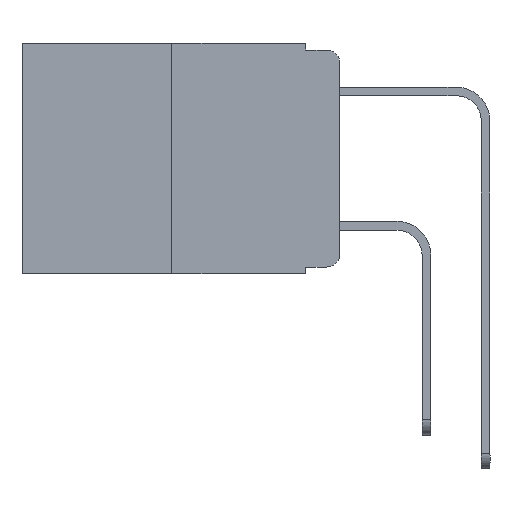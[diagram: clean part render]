
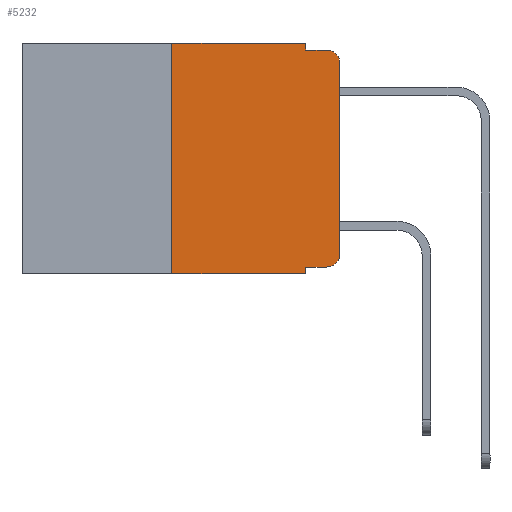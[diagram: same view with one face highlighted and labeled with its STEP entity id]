
A CAD part, left-side view. The second image highlights one B-rep face of the part: STEP entity #5232.
In plain terms, the highlighted planar face has unit normal (-1, 0, 0).
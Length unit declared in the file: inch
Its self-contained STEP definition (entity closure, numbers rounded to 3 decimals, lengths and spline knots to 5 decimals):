
#490 = AXIS2_PLACEMENT_3D ( 'NONE', #6727, #19759, #14586 ) ;
#1292 = VECTOR ( 'NONE', #14065, 39.37008 ) ;
#1585 = CARTESIAN_POINT ( 'NONE',  ( 0., 0.473, -0.343 ) ) ;
#1588 = CARTESIAN_POINT ( 'NONE',  ( 0., 0.25, 0. ) ) ;
#2134 = CARTESIAN_POINT ( 'NONE',  ( 0., 0., 0. ) ) ;
#2191 = EDGE_CURVE ( 'NONE', #2235, #18027, #21104, .T. ) ;
#2235 = VERTEX_POINT ( 'NONE', #5499 ) ;
#2695 = DIRECTION ( 'NONE',  ( 0., 0., 1. ) ) ;
#2850 = LINE ( 'NONE', #12035, #19151 ) ;
#2946 = PLANE ( 'NONE',  #490 ) ;
#3250 = VERTEX_POINT ( 'NONE', #4973 ) ;
#3470 = EDGE_CURVE ( 'NONE', #22289, #11486, #19493, .T. ) ;
#3497 = DIRECTION ( 'NONE',  ( -1., 0., 0. ) ) ;
#3571 = CARTESIAN_POINT ( 'NONE',  ( 0., 0.051, -0.333 ) ) ;
#4194 = CARTESIAN_POINT ( 'NONE',  ( 0., 0.02, -0.313 ) ) ;
#4538 = CARTESIAN_POINT ( 'NONE',  ( 0., 0.25, 0. ) ) ;
#4973 = CARTESIAN_POINT ( 'NONE',  ( 0., 0.051, 0. ) ) ;
#5232 = ADVANCED_FACE ( 'NONE', ( #16016 ), #2946, .F. ) ;
#5252 = LINE ( 'NONE', #21573, #1292 ) ;
#5464 = DIRECTION ( 'NONE',  ( 0., 0., -1. ) ) ;
#5499 = CARTESIAN_POINT ( 'NONE',  ( 0., 0.25, -0.343 ) ) ;
#6015 = VECTOR ( 'NONE', #17692, 39.37008 ) ;
#6425 = ORIENTED_EDGE ( 'NONE', *, *, #18147, .F. ) ;
#6727 = CARTESIAN_POINT ( 'NONE',  ( 0., 0.473, 0. ) ) ;
#7131 = ORIENTED_EDGE ( 'NONE', *, *, #20478, .T. ) ;
#7153 = EDGE_CURVE ( 'NONE', #15029, #11381, #17422, .T. ) ;
#7703 = DIRECTION ( 'NONE',  ( 0., 0., 1. ) ) ;
#7912 = VECTOR ( 'NONE', #12265, 39.37008 ) ;
#9179 = DIRECTION ( 'NONE',  ( 0., -1., 0. ) ) ;
#9454 = EDGE_LOOP ( 'NONE', ( #20697, #14267, #6425, #12730, #12422, #18615, #7131, #21110, #19081, #22330 ) ) ;
#10006 = EDGE_CURVE ( 'NONE', #11486, #15029, #16895, .T. ) ;
#10719 = CARTESIAN_POINT ( 'NONE',  ( 0., 0.051, -0.333 ) ) ;
#10832 = CARTESIAN_POINT ( 'NONE',  ( 0., 0.02, -0.333 ) ) ;
#11381 = VERTEX_POINT ( 'NONE', #18745 ) ;
#11486 = VERTEX_POINT ( 'NONE', #15111 ) ;
#11696 = CARTESIAN_POINT ( 'NONE',  ( 0., 0.051, -0.343 ) ) ;
#12035 = CARTESIAN_POINT ( 'NONE',  ( 0., 0.051, 0. ) ) ;
#12265 = DIRECTION ( 'NONE',  ( 0., -1., 0. ) ) ;
#12422 = ORIENTED_EDGE ( 'NONE', *, *, #13322, .F. ) ;
#12581 = VECTOR ( 'NONE', #2695, 39.37008 ) ;
#12686 = VERTEX_POINT ( 'NONE', #11696 ) ;
#12730 = ORIENTED_EDGE ( 'NONE', *, *, #18764, .F. ) ;
#13322 = EDGE_CURVE ( 'NONE', #18027, #3250, #17628, .T. ) ;
#13506 = DIRECTION ( 'NONE',  ( 0., 0., -1. ) ) ;
#13620 = DIRECTION ( 'NONE',  ( 0., 0., -1. ) ) ;
#13999 = CARTESIAN_POINT ( 'NONE',  ( 0., 0.051, -0.01 ) ) ;
#14065 = DIRECTION ( 'NONE',  ( 0., 0., -1. ) ) ;
#14105 = CARTESIAN_POINT ( 'NONE',  ( 0., 0.473, 0. ) ) ;
#14142 = LINE ( 'NONE', #10719, #18421 ) ;
#14267 = ORIENTED_EDGE ( 'NONE', *, *, #7153, .T. ) ;
#14409 = LINE ( 'NONE', #1585, #6015 ) ;
#14586 = DIRECTION ( 'NONE',  ( 0., 0., -1. ) ) ;
#14664 = CARTESIAN_POINT ( 'NONE',  ( 0., 0.051, -0.01 ) ) ;
#15027 = EDGE_CURVE ( 'NONE', #22697, #12686, #2850, .T. ) ;
#15029 = VERTEX_POINT ( 'NONE', #21139 ) ;
#15111 = CARTESIAN_POINT ( 'NONE',  ( 0., 0., -0.313 ) ) ;
#15453 = DIRECTION ( 'NONE',  ( -1., 0., 0. ) ) ;
#16016 = FACE_OUTER_BOUND ( 'NONE', #9454, .T. ) ;
#16895 = LINE ( 'NONE', #2134, #19052 ) ;
#17422 = CIRCLE ( 'NONE', #18957, 0.02 ) ;
#17628 = LINE ( 'NONE', #14105, #7912 ) ;
#17692 = DIRECTION ( 'NONE',  ( 0., -1., 0. ) ) ;
#18027 = VERTEX_POINT ( 'NONE', #1588 ) ;
#18135 = DIRECTION ( 'NONE',  ( 0., -1., 0. ) ) ;
#18147 = EDGE_CURVE ( 'NONE', #23758, #11381, #22390, .T. ) ;
#18421 = VECTOR ( 'NONE', #18135, 39.37008 ) ;
#18615 = ORIENTED_EDGE ( 'NONE', *, *, #2191, .F. ) ;
#18745 = CARTESIAN_POINT ( 'NONE',  ( 0., 0.02, -0.01 ) ) ;
#18764 = EDGE_CURVE ( 'NONE', #3250, #23758, #5252, .T. ) ;
#18957 = AXIS2_PLACEMENT_3D ( 'NONE', #20077, #3497, #5464 ) ;
#19052 = VECTOR ( 'NONE', #7703, 39.37008 ) ;
#19081 = ORIENTED_EDGE ( 'NONE', *, *, #22187, .T. ) ;
#19151 = VECTOR ( 'NONE', #13506, 39.37008 ) ;
#19493 = CIRCLE ( 'NONE', #23794, 0.02 ) ;
#19759 = DIRECTION ( 'NONE',  ( 1., 0., 0. ) ) ;
#20077 = CARTESIAN_POINT ( 'NONE',  ( 0., 0.02, -0.03 ) ) ;
#20478 = EDGE_CURVE ( 'NONE', #2235, #12686, #14409, .T. ) ;
#20697 = ORIENTED_EDGE ( 'NONE', *, *, #10006, .T. ) ;
#21104 = LINE ( 'NONE', #4538, #12581 ) ;
#21110 = ORIENTED_EDGE ( 'NONE', *, *, #15027, .F. ) ;
#21139 = CARTESIAN_POINT ( 'NONE',  ( 0., 0., -0.03 ) ) ;
#21573 = CARTESIAN_POINT ( 'NONE',  ( 0., 0.051, 0. ) ) ;
#22187 = EDGE_CURVE ( 'NONE', #22697, #22289, #14142, .T. ) ;
#22289 = VERTEX_POINT ( 'NONE', #10832 ) ;
#22330 = ORIENTED_EDGE ( 'NONE', *, *, #3470, .T. ) ;
#22390 = LINE ( 'NONE', #14664, #22578 ) ;
#22578 = VECTOR ( 'NONE', #9179, 39.37008 ) ;
#22697 = VERTEX_POINT ( 'NONE', #3571 ) ;
#23758 = VERTEX_POINT ( 'NONE', #13999 ) ;
#23794 = AXIS2_PLACEMENT_3D ( 'NONE', #4194, #15453, #13620 ) ;
